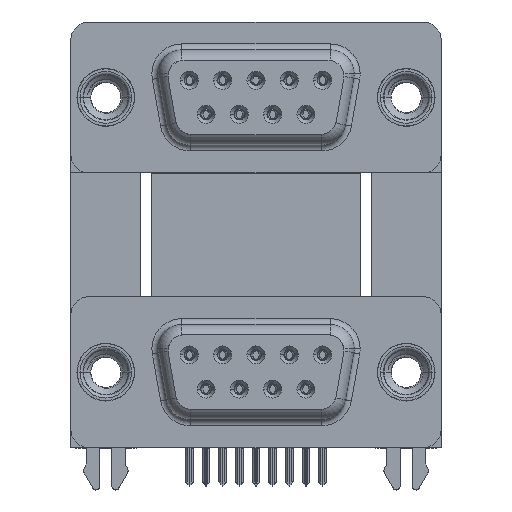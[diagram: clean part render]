
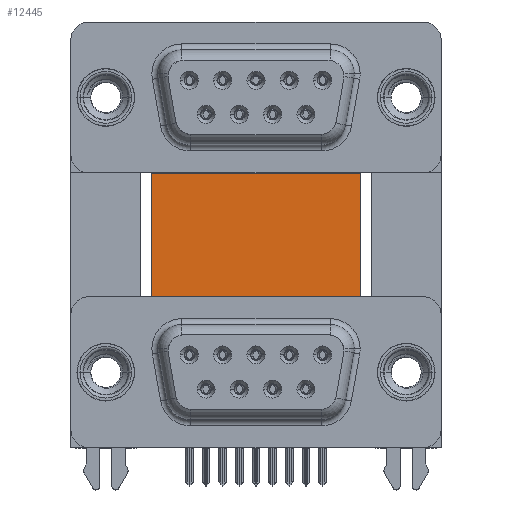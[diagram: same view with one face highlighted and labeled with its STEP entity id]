
A CAD part, top view. The second image highlights one B-rep face of the part: STEP entity #12445.
In plain terms, the highlighted planar face has unit normal (0, 0, 1).
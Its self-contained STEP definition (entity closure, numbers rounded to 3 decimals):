
#246 = LINE ( 'NONE', #9970, #9241 ) ;
#629 = DIRECTION ( 'NONE',  ( 0., 1., 0. ) ) ;
#1645 = CARTESIAN_POINT ( 'NONE',  ( 3.79, -0.735, -12. ) ) ;
#2048 = LINE ( 'NONE', #36627, #23082 ) ;
#2898 = DIRECTION ( 'NONE',  ( 0., -1., 0. ) ) ;
#3968 = EDGE_CURVE ( 'NONE', #5853, #11700, #8620, .T. ) ;
#4596 = CARTESIAN_POINT ( 'NONE',  ( 3.79, 16.585, -12. ) ) ;
#5243 = DIRECTION ( 'NONE',  ( 1., 0., 0. ) ) ;
#5853 = VERTEX_POINT ( 'NONE', #38385 ) ;
#7662 = CARTESIAN_POINT ( 'NONE',  ( 3.79, 16.585, -12. ) ) ;
#8620 = LINE ( 'NONE', #22425, #43847 ) ;
#8954 = EDGE_CURVE ( 'NONE', #42759, #19213, #9538, .T. ) ;
#9241 = VECTOR ( 'NONE', #35046, 1000. ) ;
#9538 = LINE ( 'NONE', #41196, #36668 ) ;
#9970 = CARTESIAN_POINT ( 'NONE',  ( 22.09, -3.735, -12. ) ) ;
#10012 = ORIENTED_EDGE ( 'NONE', *, *, #18258, .T. ) ;
#10068 = CARTESIAN_POINT ( 'NONE',  ( 22.59, -4.635, -12. ) ) ;
#10322 = CARTESIAN_POINT ( 'NONE',  ( 21.2, 16.585, -12. ) ) ;
#10402 = ORIENTED_EDGE ( 'NONE', *, *, #11238, .T. ) ;
#11238 = EDGE_CURVE ( 'NONE', #27283, #32012, #34850, .T. ) ;
#11700 = VERTEX_POINT ( 'NONE', #10068 ) ;
#12107 = DIRECTION ( 'NONE',  ( -0.336, -0.942, 0. ) ) ;
#12185 = CARTESIAN_POINT ( 'NONE',  ( 21.2, 16.585, -12. ) ) ;
#12415 = DIRECTION ( 'NONE',  ( 0., 0., -1. ) ) ;
#12445 = ADVANCED_FACE ( 'NONE', ( #15795 ), #29842, .F. ) ;
#14095 = ORIENTED_EDGE ( 'NONE', *, *, #21854, .T. ) ;
#14396 = VECTOR ( 'NONE', #31677, 1000. ) ;
#14670 = LINE ( 'NONE', #7662, #38737 ) ;
#15279 = CARTESIAN_POINT ( 'NONE',  ( 2.4, -4.635, -12. ) ) ;
#15492 = CARTESIAN_POINT ( 'NONE',  ( 2.9, -4.635, -12. ) ) ;
#15676 = VERTEX_POINT ( 'NONE', #18992 ) ;
#15795 = FACE_OUTER_BOUND ( 'NONE', #37225, .T. ) ;
#16036 = DIRECTION ( 'NONE',  ( -0.336, 0.942, 0. ) ) ;
#17431 = VERTEX_POINT ( 'NONE', #34638 ) ;
#18258 = EDGE_CURVE ( 'NONE', #42759, #38072, #14670, .T. ) ;
#18992 = CARTESIAN_POINT ( 'NONE',  ( 2.9, -4.635, -12. ) ) ;
#19213 = VERTEX_POINT ( 'NONE', #12185 ) ;
#19423 = DIRECTION ( 'NONE',  ( -1., 0., 0. ) ) ;
#19564 = ORIENTED_EDGE ( 'NONE', *, *, #19944, .T. ) ;
#19828 = ORIENTED_EDGE ( 'NONE', *, *, #42101, .F. ) ;
#19944 = EDGE_CURVE ( 'NONE', #32012, #5853, #246, .T. ) ;
#20020 = VECTOR ( 'NONE', #629, 1000. ) ;
#20095 = CARTESIAN_POINT ( 'NONE',  ( 3.79, 16.585, -12. ) ) ;
#21499 = CARTESIAN_POINT ( 'NONE',  ( 3.79, -3.735, -12. ) ) ;
#21854 = EDGE_CURVE ( 'NONE', #11700, #28234, #2048, .T. ) ;
#22425 = CARTESIAN_POINT ( 'NONE',  ( 22.09, -4.635, -12. ) ) ;
#22669 = ORIENTED_EDGE ( 'NONE', *, *, #38451, .T. ) ;
#23082 = VECTOR ( 'NONE', #16036, 1000. ) ;
#24144 = CARTESIAN_POINT ( 'NONE',  ( 2.9, -3.735, -12. ) ) ;
#25019 = VECTOR ( 'NONE', #25923, 1000. ) ;
#25923 = DIRECTION ( 'NONE',  ( 1., 0., 0. ) ) ;
#26033 = VECTOR ( 'NONE', #2898, 1000. ) ;
#27283 = VERTEX_POINT ( 'NONE', #33171 ) ;
#27299 = LINE ( 'NONE', #10322, #26033 ) ;
#27990 = LINE ( 'NONE', #24144, #20020 ) ;
#28234 = VERTEX_POINT ( 'NONE', #28765 ) ;
#28477 = DIRECTION ( 'NONE',  ( 0., -1., 0. ) ) ;
#28765 = CARTESIAN_POINT ( 'NONE',  ( 21.2, -0.735, -12. ) ) ;
#29842 = PLANE ( 'NONE',  #42917 ) ;
#31677 = DIRECTION ( 'NONE',  ( 1., 0., 0. ) ) ;
#32012 = VERTEX_POINT ( 'NONE', #36705 ) ;
#32707 = LINE ( 'NONE', #15279, #43861 ) ;
#32787 = ORIENTED_EDGE ( 'NONE', *, *, #3968, .T. ) ;
#33171 = CARTESIAN_POINT ( 'NONE',  ( 2.9, -3.735, -12. ) ) ;
#33502 = DIRECTION ( 'NONE',  ( 1., 0., 0. ) ) ;
#34487 = EDGE_CURVE ( 'NONE', #17431, #15676, #36323, .T. ) ;
#34542 = EDGE_CURVE ( 'NONE', #38072, #17431, #32707, .T. ) ;
#34638 = CARTESIAN_POINT ( 'NONE',  ( 2.4, -4.635, -12. ) ) ;
#34850 = LINE ( 'NONE', #21499, #14396 ) ;
#35046 = DIRECTION ( 'NONE',  ( 0., -1., 0. ) ) ;
#36046 = ORIENTED_EDGE ( 'NONE', *, *, #34487, .T. ) ;
#36323 = LINE ( 'NONE', #15492, #25019 ) ;
#36627 = CARTESIAN_POINT ( 'NONE',  ( 22.59, -4.635, -12. ) ) ;
#36668 = VECTOR ( 'NONE', #33502, 1000. ) ;
#36705 = CARTESIAN_POINT ( 'NONE',  ( 22.09, -3.735, -12. ) ) ;
#37225 = EDGE_LOOP ( 'NONE', ( #10402, #19564, #32787, #14095, #19828, #39161, #10012, #39147, #36046, #22669 ) ) ;
#38072 = VERTEX_POINT ( 'NONE', #1645 ) ;
#38385 = CARTESIAN_POINT ( 'NONE',  ( 22.09, -4.635, -12. ) ) ;
#38451 = EDGE_CURVE ( 'NONE', #15676, #27283, #27990, .T. ) ;
#38737 = VECTOR ( 'NONE', #28477, 1000. ) ;
#39147 = ORIENTED_EDGE ( 'NONE', *, *, #34542, .T. ) ;
#39161 = ORIENTED_EDGE ( 'NONE', *, *, #8954, .F. ) ;
#41196 = CARTESIAN_POINT ( 'NONE',  ( 3.79, 16.585, -12. ) ) ;
#42101 = EDGE_CURVE ( 'NONE', #19213, #28234, #27299, .T. ) ;
#42759 = VERTEX_POINT ( 'NONE', #4596 ) ;
#42917 = AXIS2_PLACEMENT_3D ( 'NONE', #20095, #12415, #19423 ) ;
#43847 = VECTOR ( 'NONE', #5243, 1000. ) ;
#43861 = VECTOR ( 'NONE', #12107, 1000. ) ;
